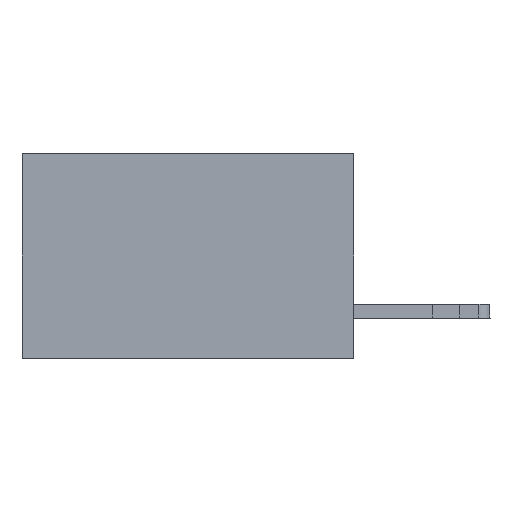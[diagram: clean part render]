
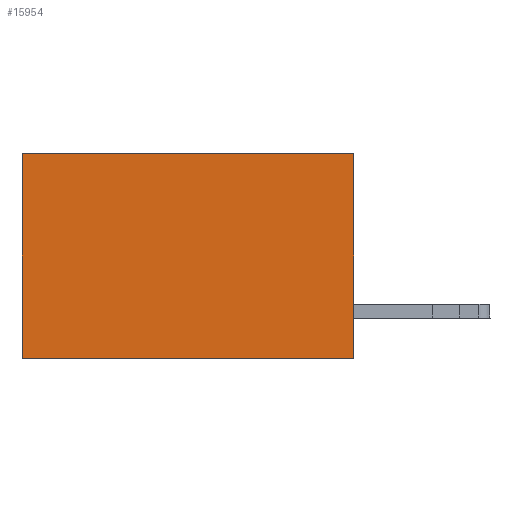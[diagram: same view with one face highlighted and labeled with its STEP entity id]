
A CAD part, left-side view. The second image highlights one B-rep face of the part: STEP entity #15954.
In plain terms, the highlighted planar face has unit normal (-1, 0, 0).
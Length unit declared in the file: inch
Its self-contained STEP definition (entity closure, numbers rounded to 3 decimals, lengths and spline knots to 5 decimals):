
#378 = ORIENTED_EDGE ( 'NONE', *, *, #12829, .F. ) ;
#1332 = VERTEX_POINT ( 'NONE', #18264 ) ;
#1573 = VERTEX_POINT ( 'NONE', #19268 ) ;
#1713 = VERTEX_POINT ( 'NONE', #12428 ) ;
#4035 = DIRECTION ( 'NONE',  ( 1., 0., 0. ) ) ;
#4733 = ORIENTED_EDGE ( 'NONE', *, *, #14949, .T. ) ;
#4917 = DIRECTION ( 'NONE',  ( 0., 1., 0. ) ) ;
#6779 = VECTOR ( 'NONE', #16196, 39.37008 ) ;
#7018 = PLANE ( 'NONE',  #11985 ) ;
#7304 = EDGE_CURVE ( 'NONE', #9205, #1713, #8239, .T. ) ;
#8239 = LINE ( 'NONE', #11272, #18173 ) ;
#9205 = VERTEX_POINT ( 'NONE', #11411 ) ;
#9876 = ORIENTED_EDGE ( 'NONE', *, *, #7304, .T. ) ;
#10969 = LINE ( 'NONE', #16949, #15946 ) ;
#11251 = EDGE_LOOP ( 'NONE', ( #4733, #378, #17505, #9876 ) ) ;
#11272 = CARTESIAN_POINT ( 'NONE',  ( 0.2875, 0., 0. ) ) ;
#11411 = CARTESIAN_POINT ( 'NONE',  ( 0.2875, 0., 0. ) ) ;
#11477 = CARTESIAN_POINT ( 'NONE',  ( 0.2875, 0., 0. ) ) ;
#11598 = CARTESIAN_POINT ( 'NONE',  ( 0.2875, 0., 0. ) ) ;
#11651 = EDGE_CURVE ( 'NONE', #9205, #1573, #16222, .T. ) ;
#11985 = AXIS2_PLACEMENT_3D ( 'NONE', #11598, #4035, #14657 ) ;
#12428 = CARTESIAN_POINT ( 'NONE',  ( 0.2875, 0.6, 0. ) ) ;
#12829 = EDGE_CURVE ( 'NONE', #1573, #1332, #10969, .T. ) ;
#13642 = VECTOR ( 'NONE', #18857, 39.37008 ) ;
#14657 = DIRECTION ( 'NONE',  ( 0., 0., -1. ) ) ;
#14765 = CARTESIAN_POINT ( 'NONE',  ( 0.2875, 0.6, 0. ) ) ;
#14949 = EDGE_CURVE ( 'NONE', #1713, #1332, #17419, .T. ) ;
#15946 = VECTOR ( 'NONE', #4917, 39.37008 ) ;
#15954 = ADVANCED_FACE ( 'NONE', ( #19241 ), #7018, .F. ) ;
#16196 = DIRECTION ( 'NONE',  ( 0., 0., -1. ) ) ;
#16222 = LINE ( 'NONE', #11477, #13642 ) ;
#16949 = CARTESIAN_POINT ( 'NONE',  ( 0.2875, 0., -0.37 ) ) ;
#17419 = LINE ( 'NONE', #14765, #6779 ) ;
#17505 = ORIENTED_EDGE ( 'NONE', *, *, #11651, .F. ) ;
#18173 = VECTOR ( 'NONE', #18964, 39.37008 ) ;
#18264 = CARTESIAN_POINT ( 'NONE',  ( 0.2875, 0.6, -0.37 ) ) ;
#18857 = DIRECTION ( 'NONE',  ( 0., 0., -1. ) ) ;
#18964 = DIRECTION ( 'NONE',  ( 0., 1., 0. ) ) ;
#19241 = FACE_OUTER_BOUND ( 'NONE', #11251, .T. ) ;
#19268 = CARTESIAN_POINT ( 'NONE',  ( 0.2875, 0., -0.37 ) ) ;
